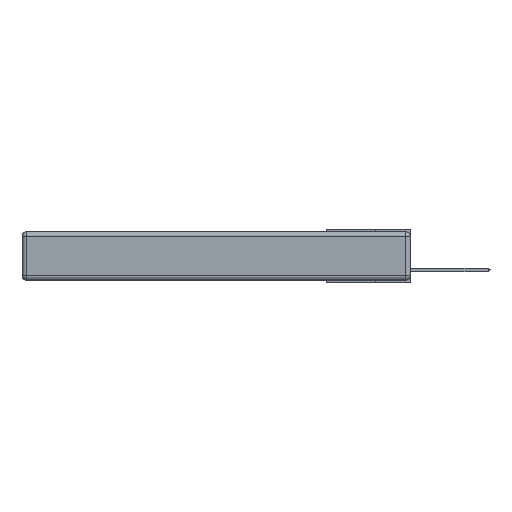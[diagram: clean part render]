
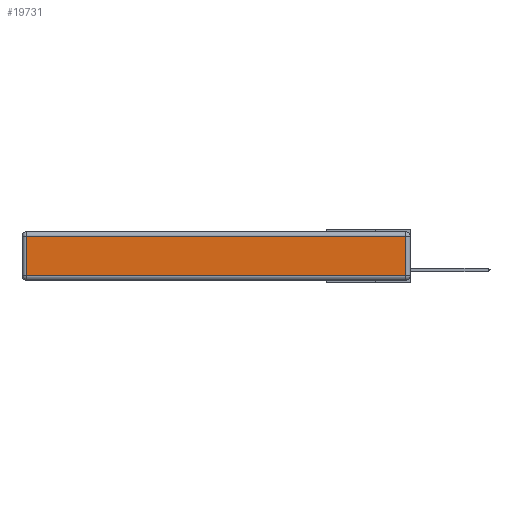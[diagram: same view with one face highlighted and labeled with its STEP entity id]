
A CAD part, left-side view. The second image highlights one B-rep face of the part: STEP entity #19731.
In plain terms, the highlighted planar face has unit normal (-1, 0, 0).
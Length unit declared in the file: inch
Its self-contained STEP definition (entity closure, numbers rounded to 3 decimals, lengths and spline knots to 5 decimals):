
#927 = CARTESIAN_POINT ( 'NONE',  ( 0., 2.72, -0.03 ) ) ;
#1529 = VERTEX_POINT ( 'NONE', #27269 ) ;
#1539 = EDGE_CURVE ( 'NONE', #3410, #13678, #25467, .T. ) ;
#2132 = CARTESIAN_POINT ( 'NONE',  ( 0., 2.75, -0.03 ) ) ;
#2296 = FACE_OUTER_BOUND ( 'NONE', #25801, .T. ) ;
#3410 = VERTEX_POINT ( 'NONE', #26109 ) ;
#3815 = LINE ( 'NONE', #21147, #22008 ) ;
#4696 = DIRECTION ( 'NONE',  ( 0., 0., -1. ) ) ;
#4933 = VECTOR ( 'NONE', #18688, 39.37008 ) ;
#6048 = EDGE_CURVE ( 'NONE', #1529, #15475, #17083, .T. ) ;
#6996 = VECTOR ( 'NONE', #4696, 39.37008 ) ;
#7382 = ORIENTED_EDGE ( 'NONE', *, *, #6048, .T. ) ;
#9428 = PLANE ( 'NONE',  #17598 ) ;
#11583 = EDGE_CURVE ( 'NONE', #13678, #1529, #3815, .T. ) ;
#11715 = CARTESIAN_POINT ( 'NONE',  ( 0., 0.03, -0.313 ) ) ;
#12731 = LINE ( 'NONE', #13294, #6996 ) ;
#13294 = CARTESIAN_POINT ( 'NONE',  ( 0., 2.72, -0.343 ) ) ;
#13678 = VERTEX_POINT ( 'NONE', #11715 ) ;
#14981 = DIRECTION ( 'NONE',  ( 0., 0., 1. ) ) ;
#15475 = VERTEX_POINT ( 'NONE', #927 ) ;
#15852 = CARTESIAN_POINT ( 'NONE',  ( 0., 0., -0.343 ) ) ;
#17083 = LINE ( 'NONE', #2132, #21408 ) ;
#17598 = AXIS2_PLACEMENT_3D ( 'NONE', #15852, #26779, #22491 ) ;
#18663 = DIRECTION ( 'NONE',  ( 0., 1., 0. ) ) ;
#18688 = DIRECTION ( 'NONE',  ( 0., -1., 0. ) ) ;
#19731 = ADVANCED_FACE ( 'NONE', ( #2296 ), #9428, .T. ) ;
#20338 = EDGE_CURVE ( 'NONE', #15475, #3410, #12731, .T. ) ;
#20891 = ORIENTED_EDGE ( 'NONE', *, *, #1539, .T. ) ;
#21147 = CARTESIAN_POINT ( 'NONE',  ( 0., 0.03, -0.343 ) ) ;
#21408 = VECTOR ( 'NONE', #18663, 39.37008 ) ;
#22008 = VECTOR ( 'NONE', #14981, 39.37008 ) ;
#22269 = ORIENTED_EDGE ( 'NONE', *, *, #11583, .T. ) ;
#22491 = DIRECTION ( 'NONE',  ( 0., 0., 1. ) ) ;
#25013 = CARTESIAN_POINT ( 'NONE',  ( 0., 0., -0.313 ) ) ;
#25467 = LINE ( 'NONE', #25013, #4933 ) ;
#25801 = EDGE_LOOP ( 'NONE', ( #20891, #22269, #7382, #26866 ) ) ;
#26109 = CARTESIAN_POINT ( 'NONE',  ( 0., 2.72, -0.313 ) ) ;
#26779 = DIRECTION ( 'NONE',  ( -1., 0., 0. ) ) ;
#26866 = ORIENTED_EDGE ( 'NONE', *, *, #20338, .T. ) ;
#27269 = CARTESIAN_POINT ( 'NONE',  ( 0., 0.03, -0.03 ) ) ;
